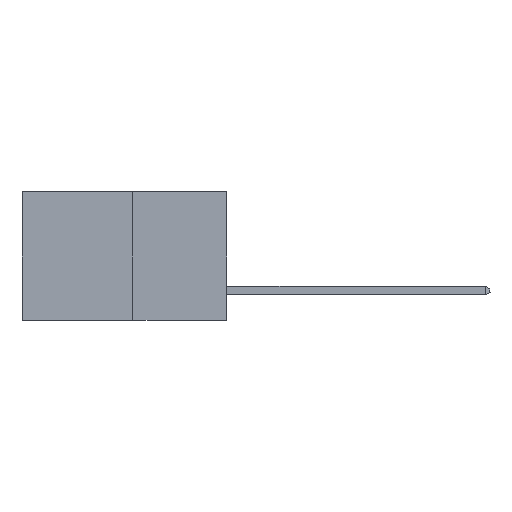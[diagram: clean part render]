
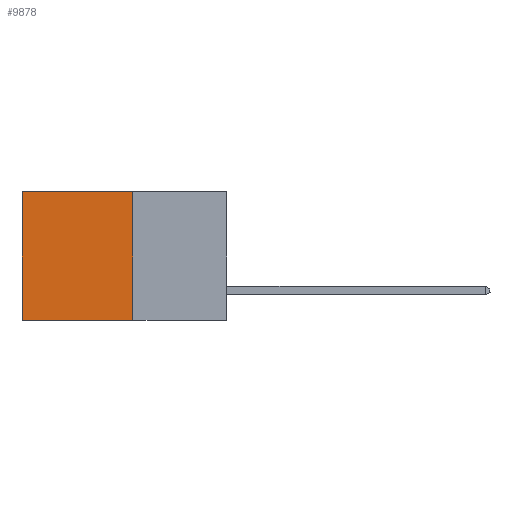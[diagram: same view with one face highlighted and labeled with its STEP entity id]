
A CAD part, left-side view. The second image highlights one B-rep face of the part: STEP entity #9878.
In plain terms, the highlighted planar face has unit normal (-1, 0, 0).
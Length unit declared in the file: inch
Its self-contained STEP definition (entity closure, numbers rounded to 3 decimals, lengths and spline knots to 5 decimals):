
#492 = VECTOR ( 'NONE', #14362, 39.37008 ) ;
#1243 = VECTOR ( 'NONE', #10828, 39.37008 ) ;
#1253 = CARTESIAN_POINT ( 'NONE',  ( 0.277, 0.59, -0.37 ) ) ;
#1887 = CARTESIAN_POINT ( 'NONE',  ( 0.277, 0.59, 0. ) ) ;
#2122 = VERTEX_POINT ( 'NONE', #16323 ) ;
#2776 = ORIENTED_EDGE ( 'NONE', *, *, #20973, .F. ) ;
#2807 = LINE ( 'NONE', #3336, #15336 ) ;
#3200 = DIRECTION ( 'NONE',  ( 0., 1., 0. ) ) ;
#3336 = CARTESIAN_POINT ( 'NONE',  ( 0.277, 0.27, 0. ) ) ;
#5303 = EDGE_CURVE ( 'NONE', #2122, #5649, #18065, .T. ) ;
#5649 = VERTEX_POINT ( 'NONE', #6807 ) ;
#5668 = PLANE ( 'NONE',  #6397 ) ;
#5864 = EDGE_CURVE ( 'NONE', #19133, #12167, #2807, .T. ) ;
#6397 = AXIS2_PLACEMENT_3D ( 'NONE', #18676, #9007, #20204 ) ;
#6807 = CARTESIAN_POINT ( 'NONE',  ( 0.277, 0.59, -0.37 ) ) ;
#7671 = VECTOR ( 'NONE', #17235, 39.37008 ) ;
#8192 = LINE ( 'NONE', #18808, #7671 ) ;
#8230 = ORIENTED_EDGE ( 'NONE', *, *, #18665, .T. ) ;
#8836 = ORIENTED_EDGE ( 'NONE', *, *, #5864, .T. ) ;
#9007 = DIRECTION ( 'NONE',  ( 1., 0., 0. ) ) ;
#9878 = ADVANCED_FACE ( 'NONE', ( #18594 ), #5668, .F. ) ;
#10615 = CARTESIAN_POINT ( 'NONE',  ( 0.277, 0.27, -0.37 ) ) ;
#10828 = DIRECTION ( 'NONE',  ( 0., 1., 0. ) ) ;
#11934 = EDGE_LOOP ( 'NONE', ( #8230, #18537, #2776, #8836 ) ) ;
#12167 = VERTEX_POINT ( 'NONE', #1887 ) ;
#14362 = DIRECTION ( 'NONE',  ( 0., 0., -1. ) ) ;
#15336 = VECTOR ( 'NONE', #3200, 39.37008 ) ;
#16323 = CARTESIAN_POINT ( 'NONE',  ( 0.277, 0.27, -0.37 ) ) ;
#17235 = DIRECTION ( 'NONE',  ( 0., 0., -1. ) ) ;
#17895 = LINE ( 'NONE', #1253, #492 ) ;
#18065 = LINE ( 'NONE', #10615, #1243 ) ;
#18537 = ORIENTED_EDGE ( 'NONE', *, *, #5303, .F. ) ;
#18594 = FACE_OUTER_BOUND ( 'NONE', #11934, .T. ) ;
#18665 = EDGE_CURVE ( 'NONE', #12167, #5649, #17895, .T. ) ;
#18676 = CARTESIAN_POINT ( 'NONE',  ( 0.277, 0.27, -0.37 ) ) ;
#18808 = CARTESIAN_POINT ( 'NONE',  ( 0.277, 0.27, -0.37 ) ) ;
#19012 = CARTESIAN_POINT ( 'NONE',  ( 0.277, 0.27, 0. ) ) ;
#19133 = VERTEX_POINT ( 'NONE', #19012 ) ;
#20204 = DIRECTION ( 'NONE',  ( 0., 0., -1. ) ) ;
#20973 = EDGE_CURVE ( 'NONE', #19133, #2122, #8192, .T. ) ;
